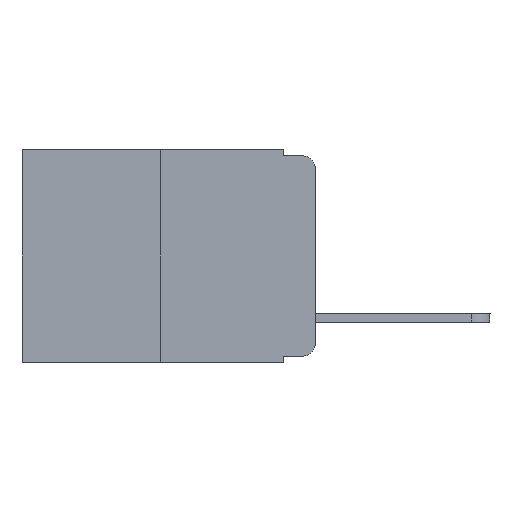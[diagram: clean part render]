
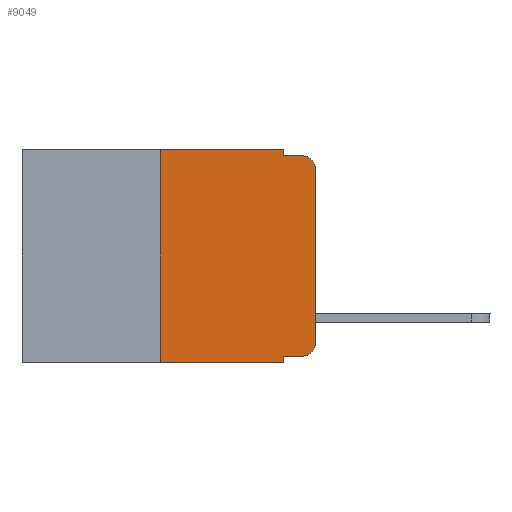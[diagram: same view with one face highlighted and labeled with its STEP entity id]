
A CAD part, left-side view. The second image highlights one B-rep face of the part: STEP entity #9049.
In plain terms, the highlighted planar face has unit normal (-1, 0, 0).
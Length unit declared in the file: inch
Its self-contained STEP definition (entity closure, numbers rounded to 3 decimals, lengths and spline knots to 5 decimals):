
#24 = VECTOR ( 'NONE', #21180, 39.37008 ) ;
#204 = LINE ( 'NONE', #18601, #5580 ) ;
#445 = CARTESIAN_POINT ( 'NONE',  ( 0., 0.25, -0.343 ) ) ;
#585 = CARTESIAN_POINT ( 'NONE',  ( 0., 0.051, -0.01 ) ) ;
#665 = DIRECTION ( 'NONE',  ( 0., 0., -1. ) ) ;
#1054 = EDGE_CURVE ( 'NONE', #18179, #20454, #8207, .T. ) ;
#1187 = DIRECTION ( 'NONE',  ( 0., 0., 1. ) ) ;
#1357 = DIRECTION ( 'NONE',  ( 0., 0., -1. ) ) ;
#2012 = CARTESIAN_POINT ( 'NONE',  ( 0., 0.051, -0.343 ) ) ;
#2058 = VECTOR ( 'NONE', #12004, 39.37008 ) ;
#2178 = ORIENTED_EDGE ( 'NONE', *, *, #20050, .T. ) ;
#2809 = LINE ( 'NONE', #8566, #2058 ) ;
#3751 = ORIENTED_EDGE ( 'NONE', *, *, #22045, .F. ) ;
#3993 = CIRCLE ( 'NONE', #21221, 0.02 ) ;
#4087 = VECTOR ( 'NONE', #17472, 39.37008 ) ;
#4332 = FACE_OUTER_BOUND ( 'NONE', #18923, .T. ) ;
#5017 = ORIENTED_EDGE ( 'NONE', *, *, #15732, .F. ) ;
#5104 = LINE ( 'NONE', #17986, #23701 ) ;
#5109 = CIRCLE ( 'NONE', #19207, 0.02 ) ;
#5236 = VERTEX_POINT ( 'NONE', #19327 ) ;
#5580 = VECTOR ( 'NONE', #7670, 39.37008 ) ;
#6237 = CARTESIAN_POINT ( 'NONE',  ( 0., 0.473, 0. ) ) ;
#6361 = LINE ( 'NONE', #6237, #8628 ) ;
#6448 = CARTESIAN_POINT ( 'NONE',  ( 0., 0.02, -0.333 ) ) ;
#6658 = VECTOR ( 'NONE', #19422, 39.37008 ) ;
#6953 = CARTESIAN_POINT ( 'NONE',  ( 0., 0.051, -0.333 ) ) ;
#7464 = DIRECTION ( 'NONE',  ( -1., 0., 0. ) ) ;
#7670 = DIRECTION ( 'NONE',  ( 0., 0., 1. ) ) ;
#7761 = LINE ( 'NONE', #17463, #6658 ) ;
#8163 = CARTESIAN_POINT ( 'NONE',  ( 0., 0., -0.03 ) ) ;
#8207 = LINE ( 'NONE', #13966, #21577 ) ;
#8502 = VERTEX_POINT ( 'NONE', #445 ) ;
#8547 = VERTEX_POINT ( 'NONE', #8163 ) ;
#8566 = CARTESIAN_POINT ( 'NONE',  ( 0., 0.473, -0.343 ) ) ;
#8628 = VECTOR ( 'NONE', #17407, 39.37008 ) ;
#8818 = VERTEX_POINT ( 'NONE', #20519 ) ;
#9049 = ADVANCED_FACE ( 'NONE', ( #4332 ), #21130, .F. ) ;
#9106 = ORIENTED_EDGE ( 'NONE', *, *, #20382, .T. ) ;
#9535 = DIRECTION ( 'NONE',  ( -1., 0., 0. ) ) ;
#9976 = DIRECTION ( 'NONE',  ( 1., 0., 0. ) ) ;
#10587 = CARTESIAN_POINT ( 'NONE',  ( 0., 0., -0.313 ) ) ;
#11039 = VERTEX_POINT ( 'NONE', #16731 ) ;
#11187 = ORIENTED_EDGE ( 'NONE', *, *, #16826, .T. ) ;
#11690 = VERTEX_POINT ( 'NONE', #22798 ) ;
#12004 = DIRECTION ( 'NONE',  ( 0., -1., 0. ) ) ;
#12129 = DIRECTION ( 'NONE',  ( 0., -1., 0. ) ) ;
#13357 = ORIENTED_EDGE ( 'NONE', *, *, #1054, .T. ) ;
#13650 = VERTEX_POINT ( 'NONE', #2012 ) ;
#13691 = EDGE_CURVE ( 'NONE', #18179, #13650, #7761, .T. ) ;
#13966 = CARTESIAN_POINT ( 'NONE',  ( 0., 0.051, -0.333 ) ) ;
#14591 = ORIENTED_EDGE ( 'NONE', *, *, #15294, .F. ) ;
#15294 = EDGE_CURVE ( 'NONE', #5236, #11690, #6361, .T. ) ;
#15611 = EDGE_CURVE ( 'NONE', #20454, #16291, #5109, .T. ) ;
#15732 = EDGE_CURVE ( 'NONE', #8818, #11039, #21065, .T. ) ;
#16291 = VERTEX_POINT ( 'NONE', #10587 ) ;
#16731 = CARTESIAN_POINT ( 'NONE',  ( 0., 0.02, -0.01 ) ) ;
#16826 = EDGE_CURVE ( 'NONE', #8547, #11039, #3993, .T. ) ;
#16990 = CARTESIAN_POINT ( 'NONE',  ( 0., 0.051, 0. ) ) ;
#17407 = DIRECTION ( 'NONE',  ( 0., -1., 0. ) ) ;
#17463 = CARTESIAN_POINT ( 'NONE',  ( 0., 0.051, 0. ) ) ;
#17472 = DIRECTION ( 'NONE',  ( 0., 0., -1. ) ) ;
#17986 = CARTESIAN_POINT ( 'NONE',  ( 0., 0.25, 0. ) ) ;
#18179 = VERTEX_POINT ( 'NONE', #6953 ) ;
#18601 = CARTESIAN_POINT ( 'NONE',  ( 0., 0., 0. ) ) ;
#18923 = EDGE_LOOP ( 'NONE', ( #9106, #11187, #5017, #3751, #14591, #23132, #2178, #20405, #13357, #21704 ) ) ;
#19207 = AXIS2_PLACEMENT_3D ( 'NONE', #22413, #9535, #20323 ) ;
#19296 = CARTESIAN_POINT ( 'NONE',  ( 0., 0.473, 0. ) ) ;
#19327 = CARTESIAN_POINT ( 'NONE',  ( 0., 0.25, 0. ) ) ;
#19422 = DIRECTION ( 'NONE',  ( 0., 0., -1. ) ) ;
#19862 = AXIS2_PLACEMENT_3D ( 'NONE', #19296, #9976, #665 ) ;
#20050 = EDGE_CURVE ( 'NONE', #8502, #13650, #2809, .T. ) ;
#20323 = DIRECTION ( 'NONE',  ( 0., 0., -1. ) ) ;
#20382 = EDGE_CURVE ( 'NONE', #16291, #8547, #204, .T. ) ;
#20405 = ORIENTED_EDGE ( 'NONE', *, *, #13691, .F. ) ;
#20454 = VERTEX_POINT ( 'NONE', #6448 ) ;
#20519 = CARTESIAN_POINT ( 'NONE',  ( 0., 0.051, -0.01 ) ) ;
#20661 = LINE ( 'NONE', #16990, #4087 ) ;
#21065 = LINE ( 'NONE', #585, #24 ) ;
#21130 = PLANE ( 'NONE',  #19862 ) ;
#21180 = DIRECTION ( 'NONE',  ( 0., -1., 0. ) ) ;
#21221 = AXIS2_PLACEMENT_3D ( 'NONE', #22085, #7464, #1357 ) ;
#21577 = VECTOR ( 'NONE', #12129, 39.37008 ) ;
#21704 = ORIENTED_EDGE ( 'NONE', *, *, #15611, .T. ) ;
#22045 = EDGE_CURVE ( 'NONE', #11690, #8818, #20661, .T. ) ;
#22085 = CARTESIAN_POINT ( 'NONE',  ( 0., 0.02, -0.03 ) ) ;
#22413 = CARTESIAN_POINT ( 'NONE',  ( 0., 0.02, -0.313 ) ) ;
#22798 = CARTESIAN_POINT ( 'NONE',  ( 0., 0.051, 0. ) ) ;
#23049 = EDGE_CURVE ( 'NONE', #8502, #5236, #5104, .T. ) ;
#23132 = ORIENTED_EDGE ( 'NONE', *, *, #23049, .F. ) ;
#23701 = VECTOR ( 'NONE', #1187, 39.37008 ) ;
